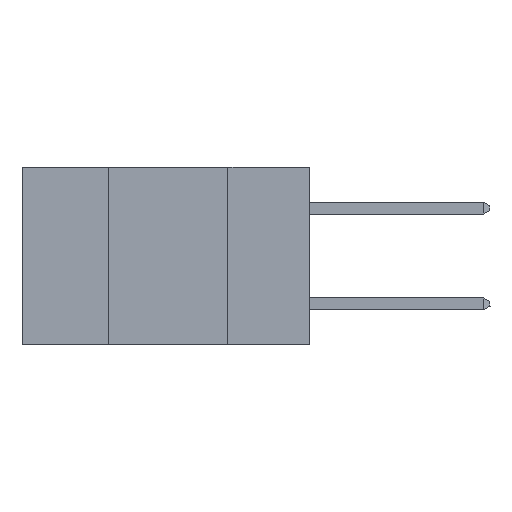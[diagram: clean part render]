
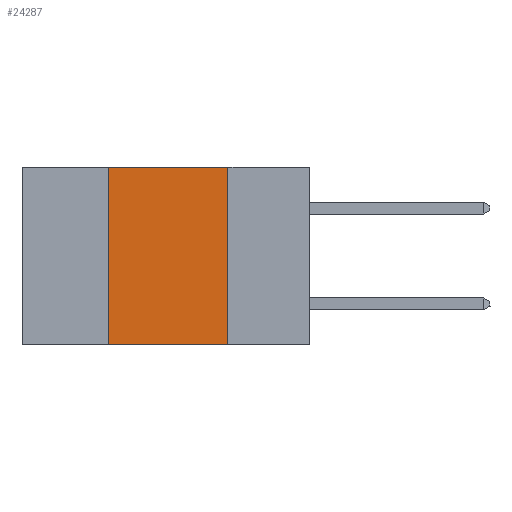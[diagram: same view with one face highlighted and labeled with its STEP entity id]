
A CAD part, left-side view. The second image highlights one B-rep face of the part: STEP entity #24287.
In plain terms, the highlighted planar face has unit normal (-1, 0, 0).
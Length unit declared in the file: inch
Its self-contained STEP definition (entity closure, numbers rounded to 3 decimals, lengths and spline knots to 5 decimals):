
#1543 = EDGE_CURVE ( 'NONE', #17132, #2100, #17963, .T. ) ;
#2100 = VERTEX_POINT ( 'NONE', #2415 ) ;
#2415 = CARTESIAN_POINT ( 'NONE',  ( 0., 0.42, 0. ) ) ;
#2766 = EDGE_LOOP ( 'NONE', ( #6976, #2941, #17338, #13099 ) ) ;
#2881 = VECTOR ( 'NONE', #26136, 39.37008 ) ;
#2941 = ORIENTED_EDGE ( 'NONE', *, *, #3703, .F. ) ;
#3703 = EDGE_CURVE ( 'NONE', #2100, #11566, #26174, .T. ) ;
#5748 = VECTOR ( 'NONE', #16304, 39.37008 ) ;
#6088 = VECTOR ( 'NONE', #10063, 39.37008 ) ;
#6115 = EDGE_CURVE ( 'NONE', #11566, #11568, #13896, .T. ) ;
#6194 = CARTESIAN_POINT ( 'NONE',  ( 0., 0.6, -0.37 ) ) ;
#6976 = ORIENTED_EDGE ( 'NONE', *, *, #6115, .F. ) ;
#8472 = DIRECTION ( 'NONE',  ( 0., 0., -1. ) ) ;
#10009 = CARTESIAN_POINT ( 'NONE',  ( 0., 0.6, 0. ) ) ;
#10063 = DIRECTION ( 'NONE',  ( 0., -1., 0. ) ) ;
#11192 = CARTESIAN_POINT ( 'NONE',  ( 0., 0.17, -0.37 ) ) ;
#11566 = VERTEX_POINT ( 'NONE', #17616 ) ;
#11568 = VERTEX_POINT ( 'NONE', #11192 ) ;
#12885 = VECTOR ( 'NONE', #18480, 39.37008 ) ;
#13099 = ORIENTED_EDGE ( 'NONE', *, *, #19760, .T. ) ;
#13896 = LINE ( 'NONE', #23872, #2881 ) ;
#14230 = CARTESIAN_POINT ( 'NONE',  ( 0., 0.42, 0. ) ) ;
#16304 = DIRECTION ( 'NONE',  ( 0., -1., 0. ) ) ;
#17132 = VERTEX_POINT ( 'NONE', #19660 ) ;
#17338 = ORIENTED_EDGE ( 'NONE', *, *, #1543, .F. ) ;
#17616 = CARTESIAN_POINT ( 'NONE',  ( 0., 0.17, 0. ) ) ;
#17963 = LINE ( 'NONE', #14230, #12885 ) ;
#18480 = DIRECTION ( 'NONE',  ( 0., 0., 1. ) ) ;
#18647 = DIRECTION ( 'NONE',  ( 1., 0., 0. ) ) ;
#19660 = CARTESIAN_POINT ( 'NONE',  ( 0., 0.42, -0.37 ) ) ;
#19760 = EDGE_CURVE ( 'NONE', #17132, #11568, #26364, .T. ) ;
#22373 = PLANE ( 'NONE',  #23356 ) ;
#22632 = CARTESIAN_POINT ( 'NONE',  ( 0., 0.6, 0. ) ) ;
#23356 = AXIS2_PLACEMENT_3D ( 'NONE', #22632, #18647, #8472 ) ;
#23872 = CARTESIAN_POINT ( 'NONE',  ( 0., 0.17, 0. ) ) ;
#24287 = ADVANCED_FACE ( 'NONE', ( #24908 ), #22373, .F. ) ;
#24908 = FACE_OUTER_BOUND ( 'NONE', #2766, .T. ) ;
#26136 = DIRECTION ( 'NONE',  ( 0., 0., -1. ) ) ;
#26174 = LINE ( 'NONE', #10009, #5748 ) ;
#26364 = LINE ( 'NONE', #6194, #6088 ) ;
